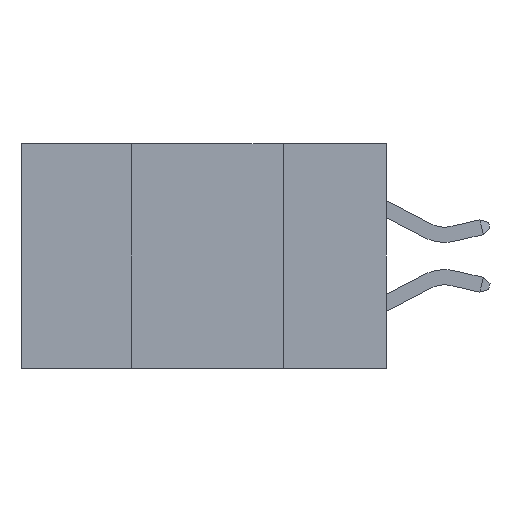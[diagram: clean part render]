
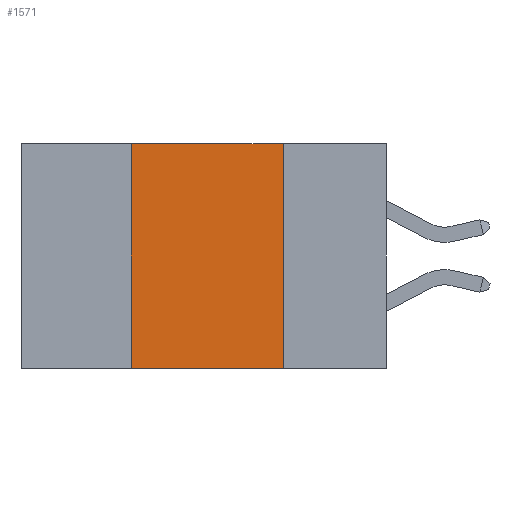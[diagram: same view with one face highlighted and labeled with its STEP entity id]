
A CAD part, left-side view. The second image highlights one B-rep face of the part: STEP entity #1571.
In plain terms, the highlighted planar face has unit normal (-1, 0, 0).
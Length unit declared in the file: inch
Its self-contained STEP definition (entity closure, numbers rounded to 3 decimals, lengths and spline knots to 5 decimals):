
#52 = LINE ( 'NONE', #2119, #2024 ) ;
#104 = EDGE_CURVE ( 'NONE', #10262, #6892, #1941, .T. ) ;
#130 = ORIENTED_EDGE ( 'NONE', *, *, #1368, .F. ) ;
#143 = DIRECTION ( 'NONE',  ( 0., -1., 0. ) ) ;
#208 = ORIENTED_EDGE ( 'NONE', *, *, #703, .F. ) ;
#349 = ORIENTED_EDGE ( 'NONE', *, *, #104, .F. ) ;
#672 = DIRECTION ( 'NONE',  ( 1., 0., 0. ) ) ;
#703 = EDGE_CURVE ( 'NONE', #6892, #6538, #9217, .T. ) ;
#829 = ORIENTED_EDGE ( 'NONE', *, *, #10561, .T. ) ;
#1304 = CARTESIAN_POINT ( 'NONE',  ( 0., 0.42, 0. ) ) ;
#1368 = EDGE_CURVE ( 'NONE', #6538, #9250, #6948, .T. ) ;
#1571 = ADVANCED_FACE ( 'NONE', ( #9300 ), #4846, .F. ) ;
#1692 = DIRECTION ( 'NONE',  ( 0., 0., -1. ) ) ;
#1941 = LINE ( 'NONE', #3522, #6329 ) ;
#2024 = VECTOR ( 'NONE', #6471, 39.37008 ) ;
#2119 = CARTESIAN_POINT ( 'NONE',  ( 0., 0.6, -0.37 ) ) ;
#2398 = VECTOR ( 'NONE', #1692, 39.37008 ) ;
#2622 = CARTESIAN_POINT ( 'NONE',  ( 0., 0.42, -0.37 ) ) ;
#3203 = CARTESIAN_POINT ( 'NONE',  ( 0., 0.17, -0.37 ) ) ;
#3522 = CARTESIAN_POINT ( 'NONE',  ( 0., 0.42, -0.37 ) ) ;
#4226 = CARTESIAN_POINT ( 'NONE',  ( 0., 0.6, 0. ) ) ;
#4846 = PLANE ( 'NONE',  #5638 ) ;
#5150 = DIRECTION ( 'NONE',  ( 0., 0., -1. ) ) ;
#5414 = CARTESIAN_POINT ( 'NONE',  ( 0., 0.17, 0. ) ) ;
#5638 = AXIS2_PLACEMENT_3D ( 'NONE', #4226, #672, #5150 ) ;
#6229 = DIRECTION ( 'NONE',  ( 0., 0., 1. ) ) ;
#6329 = VECTOR ( 'NONE', #6229, 39.37008 ) ;
#6471 = DIRECTION ( 'NONE',  ( 0., -1., 0. ) ) ;
#6538 = VERTEX_POINT ( 'NONE', #5414 ) ;
#6633 = CARTESIAN_POINT ( 'NONE',  ( 0., 0.17, -0.37 ) ) ;
#6892 = VERTEX_POINT ( 'NONE', #1304 ) ;
#6948 = LINE ( 'NONE', #3203, #2398 ) ;
#8744 = VECTOR ( 'NONE', #143, 39.37008 ) ;
#9082 = CARTESIAN_POINT ( 'NONE',  ( 0., 0.6, 0. ) ) ;
#9217 = LINE ( 'NONE', #9082, #8744 ) ;
#9250 = VERTEX_POINT ( 'NONE', #6633 ) ;
#9256 = EDGE_LOOP ( 'NONE', ( #130, #208, #349, #829 ) ) ;
#9300 = FACE_OUTER_BOUND ( 'NONE', #9256, .T. ) ;
#10262 = VERTEX_POINT ( 'NONE', #2622 ) ;
#10561 = EDGE_CURVE ( 'NONE', #10262, #9250, #52, .T. ) ;
